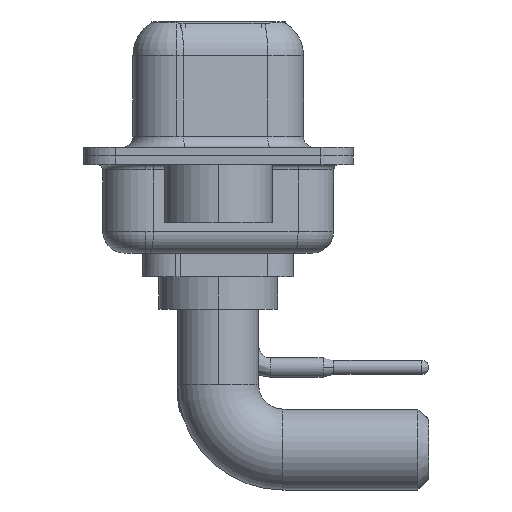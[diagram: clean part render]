
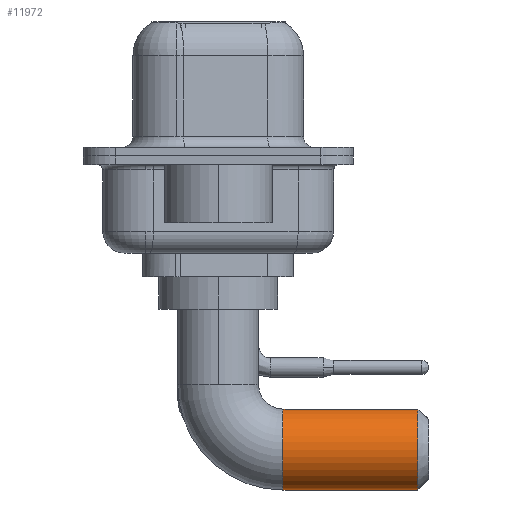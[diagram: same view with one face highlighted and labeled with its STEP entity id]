
A CAD part, left-side view. The second image highlights one B-rep face of the part: STEP entity #11972.
In plain terms, the highlighted cylindrical face has radius 1.875 mm (diameter 3.75 mm), a partial arc.
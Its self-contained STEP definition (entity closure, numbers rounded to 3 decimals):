
#635 = VERTEX_POINT ( 'NONE', #1922 ) ;
#807 = CARTESIAN_POINT ( 'NONE',  ( 0., -9.25, -4.625 ) ) ;
#870 = CARTESIAN_POINT ( 'NONE',  ( 0., -9.25, -8.375 ) ) ;
#1092 = EDGE_LOOP ( 'NONE', ( #12154, #9413, #16884, #6087 ) ) ;
#1249 = CARTESIAN_POINT ( 'NONE',  ( 0., -3., -8.375 ) ) ;
#1474 = DIRECTION ( 'NONE',  ( 0., 0., -1. ) ) ;
#1533 = DIRECTION ( 'NONE',  ( -1., 0., 0. ) ) ;
#1922 = CARTESIAN_POINT ( 'NONE',  ( 0., -3., -4.625 ) ) ;
#2682 = EDGE_CURVE ( 'NONE', #17333, #15334, #9395, .T. ) ;
#2783 = DIRECTION ( 'NONE',  ( 0., -1., 0. ) ) ;
#3574 = LINE ( 'NONE', #10354, #5688 ) ;
#4628 = VERTEX_POINT ( 'NONE', #807 ) ;
#5215 = CARTESIAN_POINT ( 'NONE',  ( 0., -3., -6.5 ) ) ;
#5688 = VECTOR ( 'NONE', #6816, 1000. ) ;
#6020 = CARTESIAN_POINT ( 'NONE',  ( 0., -3., -6.5 ) ) ;
#6087 = ORIENTED_EDGE ( 'NONE', *, *, #10432, .T. ) ;
#6170 = CIRCLE ( 'NONE', #12561, 1.875 ) ;
#6609 = DIRECTION ( 'NONE',  ( 0., 1., 0. ) ) ;
#6816 = DIRECTION ( 'NONE',  ( 0., -1., 0. ) ) ;
#9395 = LINE ( 'NONE', #14522, #15672 ) ;
#9413 = ORIENTED_EDGE ( 'NONE', *, *, #13201, .T. ) ;
#10354 = CARTESIAN_POINT ( 'NONE',  ( 0., -3., -4.625 ) ) ;
#10432 = EDGE_CURVE ( 'NONE', #15334, #4628, #6170, .T. ) ;
#11620 = AXIS2_PLACEMENT_3D ( 'NONE', #5215, #13438, #1533 ) ;
#11972 = ADVANCED_FACE ( 'NONE', ( #12911 ), #21348, .T. ) ;
#12154 = ORIENTED_EDGE ( 'NONE', *, *, #16027, .F. ) ;
#12561 = AXIS2_PLACEMENT_3D ( 'NONE', #20361, #6609, #1474 ) ;
#12911 = FACE_OUTER_BOUND ( 'NONE', #1092, .T. ) ;
#13201 = EDGE_CURVE ( 'NONE', #635, #17333, #15888, .T. ) ;
#13438 = DIRECTION ( 'NONE',  ( 0., -1., 0. ) ) ;
#14522 = CARTESIAN_POINT ( 'NONE',  ( 0., -3., -8.375 ) ) ;
#15334 = VERTEX_POINT ( 'NONE', #870 ) ;
#15672 = VECTOR ( 'NONE', #21291, 1000. ) ;
#15888 = CIRCLE ( 'NONE', #11620, 1.875 ) ;
#16027 = EDGE_CURVE ( 'NONE', #635, #4628, #3574, .T. ) ;
#16884 = ORIENTED_EDGE ( 'NONE', *, *, #2682, .T. ) ;
#17333 = VERTEX_POINT ( 'NONE', #1249 ) ;
#19076 = AXIS2_PLACEMENT_3D ( 'NONE', #6020, #2783, #21232 ) ;
#20361 = CARTESIAN_POINT ( 'NONE',  ( 0., -9.25, -6.5 ) ) ;
#21232 = DIRECTION ( 'NONE',  ( 0., 0., -1. ) ) ;
#21291 = DIRECTION ( 'NONE',  ( 0., -1., 0. ) ) ;
#21348 = CYLINDRICAL_SURFACE ( 'NONE', #19076, 1.875 ) ;
